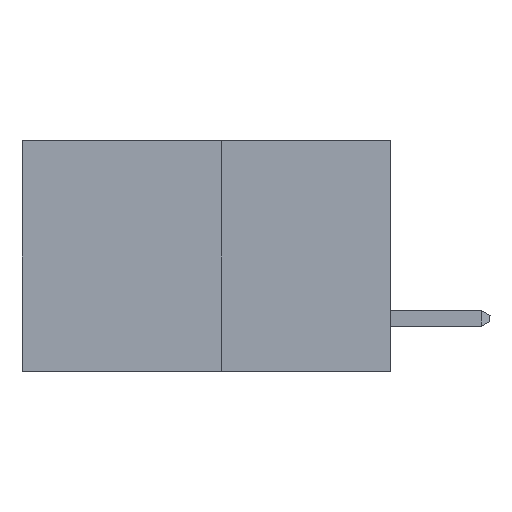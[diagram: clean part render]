
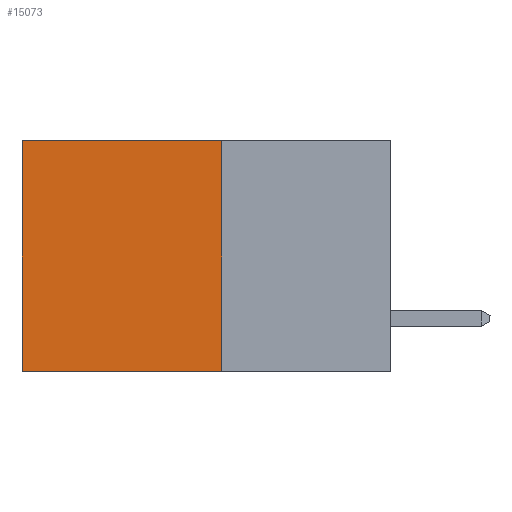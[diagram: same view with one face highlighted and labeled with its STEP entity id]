
A CAD part, left-side view. The second image highlights one B-rep face of the part: STEP entity #15073.
In plain terms, the highlighted planar face has unit normal (-1, 0, 0).
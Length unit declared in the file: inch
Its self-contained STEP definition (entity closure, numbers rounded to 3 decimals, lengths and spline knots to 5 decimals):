
#45 = ORIENTED_EDGE ( 'NONE', *, *, #25926, .F. ) ;
#1177 = EDGE_CURVE ( 'NONE', #25627, #20557, #26046, .T. ) ;
#2071 = CARTESIAN_POINT ( 'NONE',  ( 0.277, 0.59, -0.37 ) ) ;
#2157 = CARTESIAN_POINT ( 'NONE',  ( 0.277, 0.27, -0.37 ) ) ;
#2193 = DIRECTION ( 'NONE',  ( 0., 0., -1. ) ) ;
#3600 = LINE ( 'NONE', #8881, #26656 ) ;
#5414 = LINE ( 'NONE', #2071, #28106 ) ;
#7106 = CARTESIAN_POINT ( 'NONE',  ( 0.277, 0.27, -0.37 ) ) ;
#7942 = CARTESIAN_POINT ( 'NONE',  ( 0.277, 0.27, 0. ) ) ;
#8256 = VECTOR ( 'NONE', #15423, 39.37008 ) ;
#8881 = CARTESIAN_POINT ( 'NONE',  ( 0.277, 0.27, -0.37 ) ) ;
#9468 = CARTESIAN_POINT ( 'NONE',  ( 0.277, 0.59, -0.37 ) ) ;
#9850 = DIRECTION ( 'NONE',  ( 1., 0., 0. ) ) ;
#11453 = EDGE_LOOP ( 'NONE', ( #16063, #20861, #45, #15115 ) ) ;
#14265 = PLANE ( 'NONE',  #24202 ) ;
#14409 = VECTOR ( 'NONE', #15769, 39.37008 ) ;
#15073 = ADVANCED_FACE ( 'NONE', ( #21816 ), #14265, .F. ) ;
#15115 = ORIENTED_EDGE ( 'NONE', *, *, #1177, .T. ) ;
#15423 = DIRECTION ( 'NONE',  ( 0., 1., 0. ) ) ;
#15769 = DIRECTION ( 'NONE',  ( 0., 1., 0. ) ) ;
#15992 = EDGE_CURVE ( 'NONE', #23545, #22950, #26957, .T. ) ;
#16063 = ORIENTED_EDGE ( 'NONE', *, *, #23422, .T. ) ;
#16504 = CARTESIAN_POINT ( 'NONE',  ( 0.277, 0.27, -0.37 ) ) ;
#20557 = VERTEX_POINT ( 'NONE', #28456 ) ;
#20861 = ORIENTED_EDGE ( 'NONE', *, *, #15992, .F. ) ;
#21816 = FACE_OUTER_BOUND ( 'NONE', #11453, .T. ) ;
#22274 = DIRECTION ( 'NONE',  ( 0., 0., -1. ) ) ;
#22950 = VERTEX_POINT ( 'NONE', #9468 ) ;
#23422 = EDGE_CURVE ( 'NONE', #20557, #22950, #5414, .T. ) ;
#23545 = VERTEX_POINT ( 'NONE', #7106 ) ;
#24202 = AXIS2_PLACEMENT_3D ( 'NONE', #16504, #9850, #25493 ) ;
#24863 = CARTESIAN_POINT ( 'NONE',  ( 0.277, 0.27, 0. ) ) ;
#25493 = DIRECTION ( 'NONE',  ( 0., 0., -1. ) ) ;
#25627 = VERTEX_POINT ( 'NONE', #7942 ) ;
#25926 = EDGE_CURVE ( 'NONE', #25627, #23545, #3600, .T. ) ;
#26046 = LINE ( 'NONE', #24863, #8256 ) ;
#26656 = VECTOR ( 'NONE', #2193, 39.37008 ) ;
#26957 = LINE ( 'NONE', #2157, #14409 ) ;
#28106 = VECTOR ( 'NONE', #22274, 39.37008 ) ;
#28456 = CARTESIAN_POINT ( 'NONE',  ( 0.277, 0.59, 0. ) ) ;
